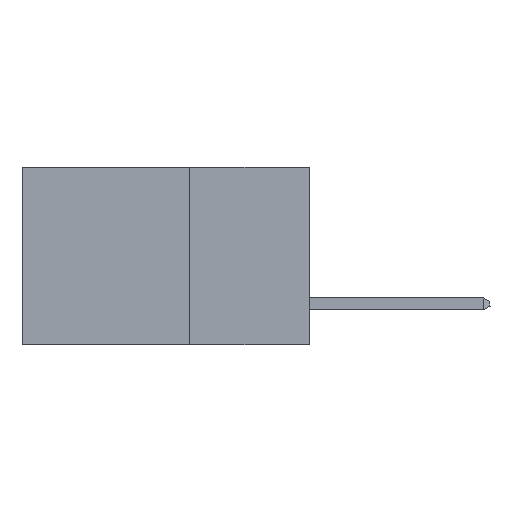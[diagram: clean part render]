
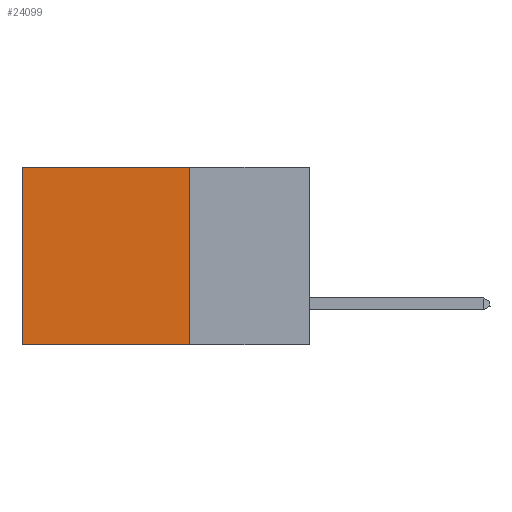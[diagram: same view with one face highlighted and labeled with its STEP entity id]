
A CAD part, left-side view. The second image highlights one B-rep face of the part: STEP entity #24099.
In plain terms, the highlighted planar face has unit normal (-1, 0, 0).
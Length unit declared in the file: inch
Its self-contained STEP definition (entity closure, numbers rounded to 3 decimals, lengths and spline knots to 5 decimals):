
#308 = DIRECTION ( 'NONE',  ( 1., 0., 0. ) ) ;
#341 = CARTESIAN_POINT ( 'NONE',  ( 0.2875, 0.25, -0.37 ) ) ;
#1834 = EDGE_CURVE ( 'NONE', #25132, #4694, #25075, .T. ) ;
#4195 = EDGE_CURVE ( 'NONE', #20286, #21289, #5804, .T. ) ;
#4694 = VERTEX_POINT ( 'NONE', #23591 ) ;
#5804 = LINE ( 'NONE', #15515, #8166 ) ;
#6274 = CARTESIAN_POINT ( 'NONE',  ( 0.2875, 0.25, 0. ) ) ;
#6371 = ORIENTED_EDGE ( 'NONE', *, *, #14243, .F. ) ;
#7237 = PLANE ( 'NONE',  #21275 ) ;
#8089 = ORIENTED_EDGE ( 'NONE', *, *, #4195, .T. ) ;
#8166 = VECTOR ( 'NONE', #17459, 39.37008 ) ;
#8802 = CARTESIAN_POINT ( 'NONE',  ( 0.2875, 0.25, 0. ) ) ;
#8899 = CARTESIAN_POINT ( 'NONE',  ( 0.2875, 0.6, 0. ) ) ;
#10827 = LINE ( 'NONE', #11045, #14426 ) ;
#11045 = CARTESIAN_POINT ( 'NONE',  ( 0.2875, 0.25, 0. ) ) ;
#11748 = DIRECTION ( 'NONE',  ( 0., 0., -1. ) ) ;
#12424 = EDGE_CURVE ( 'NONE', #21289, #4694, #20718, .T. ) ;
#14243 = EDGE_CURVE ( 'NONE', #20286, #25132, #10827, .T. ) ;
#14426 = VECTOR ( 'NONE', #19457, 39.37008 ) ;
#15043 = EDGE_LOOP ( 'NONE', ( #19414, #20905, #6371, #8089 ) ) ;
#15515 = CARTESIAN_POINT ( 'NONE',  ( 0.2875, 0.25, 0. ) ) ;
#15592 = CARTESIAN_POINT ( 'NONE',  ( 0.2875, 0.6, 0. ) ) ;
#17459 = DIRECTION ( 'NONE',  ( 0., 1., 0. ) ) ;
#19259 = DIRECTION ( 'NONE',  ( 0., 0., -1. ) ) ;
#19414 = ORIENTED_EDGE ( 'NONE', *, *, #12424, .T. ) ;
#19456 = VECTOR ( 'NONE', #21335, 39.37008 ) ;
#19457 = DIRECTION ( 'NONE',  ( 0., 0., -1. ) ) ;
#20286 = VERTEX_POINT ( 'NONE', #6274 ) ;
#20718 = LINE ( 'NONE', #8899, #24358 ) ;
#20905 = ORIENTED_EDGE ( 'NONE', *, *, #1834, .F. ) ;
#21211 = FACE_OUTER_BOUND ( 'NONE', #15043, .T. ) ;
#21275 = AXIS2_PLACEMENT_3D ( 'NONE', #8802, #308, #19259 ) ;
#21289 = VERTEX_POINT ( 'NONE', #15592 ) ;
#21335 = DIRECTION ( 'NONE',  ( 0., 1., 0. ) ) ;
#23591 = CARTESIAN_POINT ( 'NONE',  ( 0.2875, 0.6, -0.37 ) ) ;
#24099 = ADVANCED_FACE ( 'NONE', ( #21211 ), #7237, .F. ) ;
#24358 = VECTOR ( 'NONE', #11748, 39.37008 ) ;
#25075 = LINE ( 'NONE', #341, #19456 ) ;
#25132 = VERTEX_POINT ( 'NONE', #26797 ) ;
#26797 = CARTESIAN_POINT ( 'NONE',  ( 0.2875, 0.25, -0.37 ) ) ;
